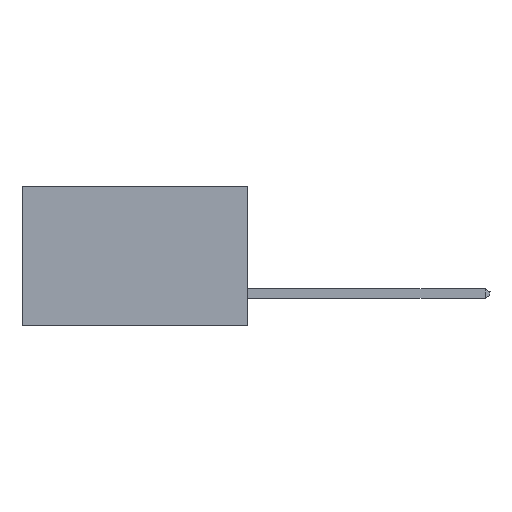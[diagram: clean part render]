
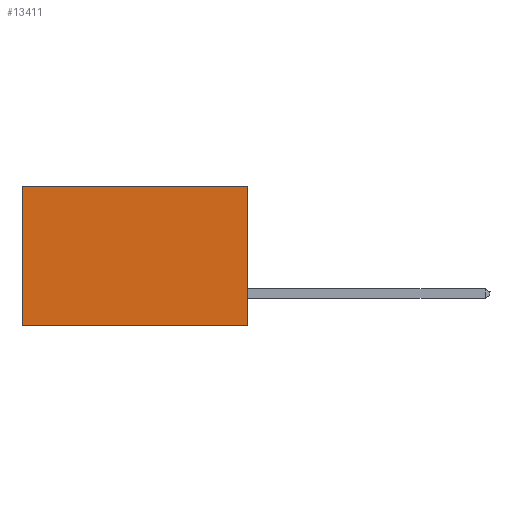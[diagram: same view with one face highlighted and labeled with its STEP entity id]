
A CAD part, left-side view. The second image highlights one B-rep face of the part: STEP entity #13411.
In plain terms, the highlighted planar face has unit normal (-1, 0, 0).
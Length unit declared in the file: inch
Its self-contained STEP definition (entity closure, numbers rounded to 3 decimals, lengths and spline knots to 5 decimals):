
#55 = ORIENTED_EDGE ( 'NONE', *, *, #15477, .T. ) ;
#470 = LINE ( 'NONE', #10273, #6569 ) ;
#508 = ORIENTED_EDGE ( 'NONE', *, *, #9896, .T. ) ;
#1017 = EDGE_LOOP ( 'NONE', ( #55, #10921, #19774, #508 ) ) ;
#1918 = DIRECTION ( 'NONE',  ( 1., 0., 0. ) ) ;
#1925 = DIRECTION ( 'NONE',  ( 0., 0., -1. ) ) ;
#2361 = DIRECTION ( 'NONE',  ( 0., 0., -1. ) ) ;
#2481 = VERTEX_POINT ( 'NONE', #10026 ) ;
#3498 = CARTESIAN_POINT ( 'NONE',  ( 0.2615, 0.6, -0.37 ) ) ;
#3895 = CARTESIAN_POINT ( 'NONE',  ( 0.2615, 0., -0.37 ) ) ;
#4004 = FACE_OUTER_BOUND ( 'NONE', #1017, .T. ) ;
#4449 = CARTESIAN_POINT ( 'NONE',  ( 0.2615, 0., -0.37 ) ) ;
#5065 = VECTOR ( 'NONE', #14018, 39.37008 ) ;
#5321 = CARTESIAN_POINT ( 'NONE',  ( 0.2615, 0., -0.37 ) ) ;
#5991 = VERTEX_POINT ( 'NONE', #7968 ) ;
#6569 = VECTOR ( 'NONE', #18518, 39.37008 ) ;
#7968 = CARTESIAN_POINT ( 'NONE',  ( 0.2615, 0., -0.37 ) ) ;
#8968 = EDGE_CURVE ( 'NONE', #16513, #5991, #17245, .T. ) ;
#9232 = LINE ( 'NONE', #4449, #20115 ) ;
#9896 = EDGE_CURVE ( 'NONE', #16513, #2481, #11054, .T. ) ;
#10026 = CARTESIAN_POINT ( 'NONE',  ( 0.2615, 0.6, 0. ) ) ;
#10273 = CARTESIAN_POINT ( 'NONE',  ( 0.2615, 0.6, -0.37 ) ) ;
#10419 = EDGE_CURVE ( 'NONE', #5991, #14004, #9232, .T. ) ;
#10921 = ORIENTED_EDGE ( 'NONE', *, *, #10419, .F. ) ;
#11054 = LINE ( 'NONE', #17523, #5065 ) ;
#13124 = VECTOR ( 'NONE', #1925, 39.37008 ) ;
#13411 = ADVANCED_FACE ( 'NONE', ( #4004 ), #17340, .F. ) ;
#14004 = VERTEX_POINT ( 'NONE', #3498 ) ;
#14018 = DIRECTION ( 'NONE',  ( 0., 1., 0. ) ) ;
#14295 = DIRECTION ( 'NONE',  ( 0., 1., 0. ) ) ;
#15477 = EDGE_CURVE ( 'NONE', #2481, #14004, #470, .T. ) ;
#16513 = VERTEX_POINT ( 'NONE', #21130 ) ;
#17245 = LINE ( 'NONE', #5321, #13124 ) ;
#17340 = PLANE ( 'NONE',  #21195 ) ;
#17523 = CARTESIAN_POINT ( 'NONE',  ( 0.2615, 0., 0. ) ) ;
#18518 = DIRECTION ( 'NONE',  ( 0., 0., -1. ) ) ;
#19774 = ORIENTED_EDGE ( 'NONE', *, *, #8968, .F. ) ;
#20115 = VECTOR ( 'NONE', #14295, 39.37008 ) ;
#21130 = CARTESIAN_POINT ( 'NONE',  ( 0.2615, 0., 0. ) ) ;
#21195 = AXIS2_PLACEMENT_3D ( 'NONE', #3895, #1918, #2361 ) ;
